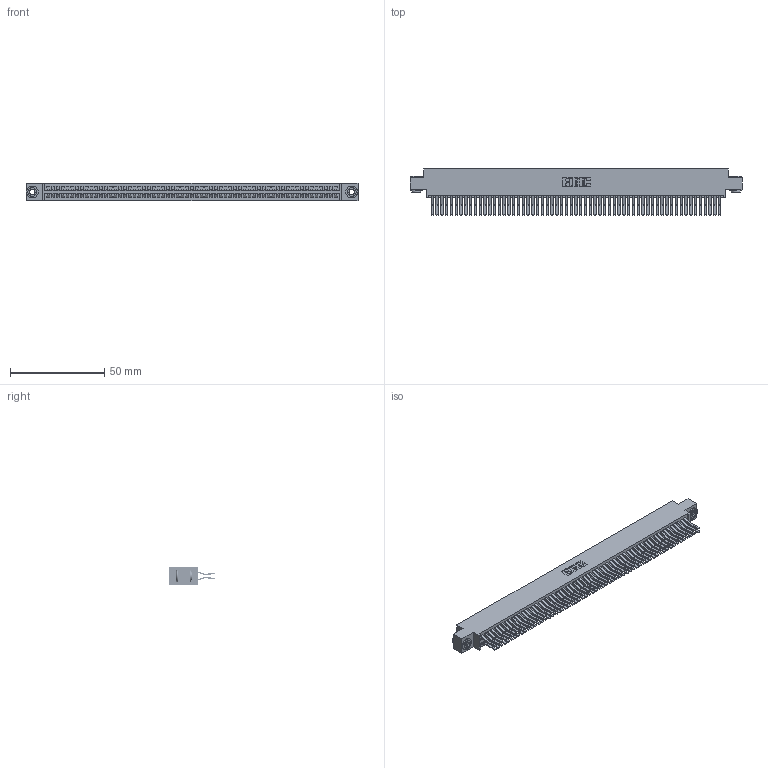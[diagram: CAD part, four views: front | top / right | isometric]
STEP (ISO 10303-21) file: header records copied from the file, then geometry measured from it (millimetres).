
FILE_DESCRIPTION (( 'STEP AP203' ), '1' );
FILE_NAME ('395-122-560-803.STEP', '2019-10-28T09:56:20', ( '' ), ( '' ), 'SwSTEP 2.0', 'SolidWorks 2016', '' );
FILE_SCHEMA (( 'CONFIG_CONTROL_DESIGN' ));
Length unit declared in the file: inch
Products named in the file (4): 345 Part_0.170 Offset - 0.156 Dia-TH; 395-122-560-803; 345-292-001_560 Tail; 345-250-002_345-250-002-102
Assembly tree (125 placements, depth 2):
  395-122-560-803
    345 Part_0.170 Offset - 0.156 Dia-TH
    345-292-001_560 Tail  x122
    345-250-002_345-250-002-102  x2
Bounding box: 176.15 x 24.45 x 9.4 mm (x, y, z)
Volume: 17993.3 mm3; surface area: 29370.2 mm2
Topology: 125 solids, 125 shells, 6512 faces, 19339 edges, 12726 vertices
Faces by surface type: plane 4120, cylinder 2384, cone 8
Entity records: 46174 total; most frequent: CARTESIAN_POINT 7699, ORIENTED_EDGE 7626, DIRECTION 6799, EDGE_CURVE 3813, LINE 3409, VECTOR 3409, VERTEX_POINT 2538, AXIS2_PLACEMENT_3D 1695
